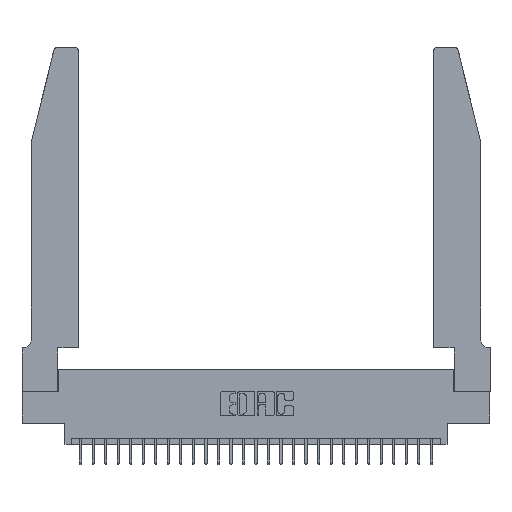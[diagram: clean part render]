
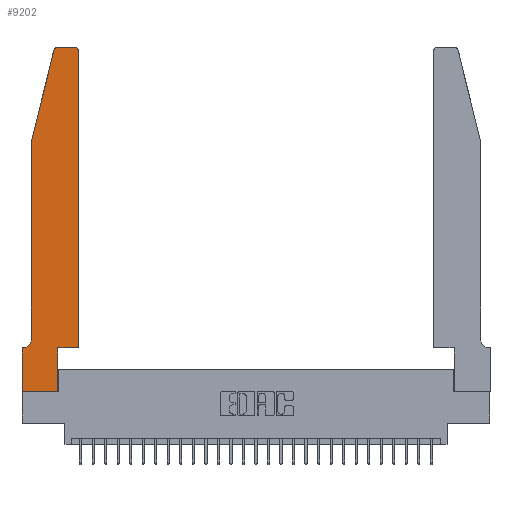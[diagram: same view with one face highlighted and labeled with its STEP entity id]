
A CAD part, top view. The second image highlights one B-rep face of the part: STEP entity #9202.
In plain terms, the highlighted planar face has unit normal (0, 0, 1).
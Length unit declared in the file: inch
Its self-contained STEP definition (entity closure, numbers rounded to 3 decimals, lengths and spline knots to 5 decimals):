
#356 = CARTESIAN_POINT ( 'NONE',  ( 0.4505, 0.35, 0.37 ) ) ;
#701 = CARTESIAN_POINT ( 'NONE',  ( 0.0755, 2., 0.37 ) ) ;
#728 = AXIS2_PLACEMENT_3D ( 'NONE', #21425, #10027, #25942 ) ;
#833 = VECTOR ( 'NONE', #1342, 39.37008 ) ;
#1273 = VECTOR ( 'NONE', #21099, 39.37008 ) ;
#1334 = CARTESIAN_POINT ( 'NONE',  ( 0.4205, 2.75, 0.37 ) ) ;
#1342 = DIRECTION ( 'NONE',  ( 0., -1., 0. ) ) ;
#1542 = EDGE_CURVE ( 'NONE', #26571, #23493, #13890, .T. ) ;
#2296 = EDGE_CURVE ( 'NONE', #9188, #12529, #13505, .T. ) ;
#2359 = ORIENTED_EDGE ( 'NONE', *, *, #21481, .T. ) ;
#2656 = CARTESIAN_POINT ( 'NONE',  ( 0.0755, 0.42, 0.37 ) ) ;
#2674 = CARTESIAN_POINT ( 'NONE',  ( 0.4505, 2.72, 0.37 ) ) ;
#2843 = CARTESIAN_POINT ( 'NONE',  ( 0.0755, 0.35, 0.37 ) ) ;
#2919 = LINE ( 'NONE', #22502, #20438 ) ;
#3110 = DIRECTION ( 'NONE',  ( 0., 1., 0. ) ) ;
#3209 = ORIENTED_EDGE ( 'NONE', *, *, #3962, .T. ) ;
#3780 = ORIENTED_EDGE ( 'NONE', *, *, #15778, .T. ) ;
#3796 = DIRECTION ( 'NONE',  ( -1., 0., 0. ) ) ;
#3881 = DIRECTION ( 'NONE',  ( -0.239, -0.971, 0. ) ) ;
#3962 = EDGE_CURVE ( 'NONE', #12656, #25117, #19539, .T. ) ;
#4898 = VERTEX_POINT ( 'NONE', #7583 ) ;
#5451 = CARTESIAN_POINT ( 'NONE',  ( 0.2865, 0., 0.37 ) ) ;
#6145 = EDGE_CURVE ( 'NONE', #12529, #4898, #19934, .T. ) ;
#6250 = FACE_OUTER_BOUND ( 'NONE', #17310, .T. ) ;
#6573 = DIRECTION ( 'NONE',  ( 0., 0., 1. ) ) ;
#6598 = LINE ( 'NONE', #2843, #18710 ) ;
#6709 = LINE ( 'NONE', #22166, #22785 ) ;
#7068 = VECTOR ( 'NONE', #18686, 39.37008 ) ;
#7450 = CARTESIAN_POINT ( 'NONE',  ( 0.0055, 0.42, 0.37 ) ) ;
#7583 = CARTESIAN_POINT ( 'NONE',  ( 0.4505, 0.35, 0.37 ) ) ;
#7631 = PLANE ( 'NONE',  #728 ) ;
#8285 = CARTESIAN_POINT ( 'NONE',  ( 0.25487, 2.72718, 0.37 ) ) ;
#8880 = EDGE_CURVE ( 'NONE', #13089, #15470, #12637, .T. ) ;
#9188 = VERTEX_POINT ( 'NONE', #5451 ) ;
#9202 = ADVANCED_FACE ( 'NONE', ( #6250 ), #7631, .T. ) ;
#9682 = VECTOR ( 'NONE', #3110, 39.37008 ) ;
#9712 = CARTESIAN_POINT ( 'NONE',  ( 0., 0., 0.37 ) ) ;
#9746 = DIRECTION ( 'NONE',  ( -1., 0., 0. ) ) ;
#9800 = ORIENTED_EDGE ( 'NONE', *, *, #8880, .T. ) ;
#9913 = CARTESIAN_POINT ( 'NONE',  ( 0.4505, 0.35, 0.37 ) ) ;
#9932 = VERTEX_POINT ( 'NONE', #8285 ) ;
#10027 = DIRECTION ( 'NONE',  ( 0., 0., 1. ) ) ;
#10673 = VECTOR ( 'NONE', #3796, 39.37008 ) ;
#10720 = AXIS2_PLACEMENT_3D ( 'NONE', #25015, #11337, #27245 ) ;
#10824 = CARTESIAN_POINT ( 'NONE',  ( 0.284, 2.75, 0.37 ) ) ;
#10858 = EDGE_CURVE ( 'NONE', #4898, #13089, #21123, .T. ) ;
#11337 = DIRECTION ( 'NONE',  ( 0., 0., 1. ) ) ;
#11508 = ORIENTED_EDGE ( 'NONE', *, *, #17144, .T. ) ;
#12090 = ORIENTED_EDGE ( 'NONE', *, *, #2296, .T. ) ;
#12384 = CARTESIAN_POINT ( 'NONE',  ( 0., 0.35, 0.37 ) ) ;
#12529 = VERTEX_POINT ( 'NONE', #14310 ) ;
#12589 = ORIENTED_EDGE ( 'NONE', *, *, #23916, .T. ) ;
#12637 = CIRCLE ( 'NONE', #24861, 0.03 ) ;
#12656 = VERTEX_POINT ( 'NONE', #12384 ) ;
#13023 = LINE ( 'NONE', #26374, #833 ) ;
#13089 = VERTEX_POINT ( 'NONE', #2674 ) ;
#13420 = EDGE_CURVE ( 'NONE', #9932, #27993, #6709, .T. ) ;
#13505 = LINE ( 'NONE', #21193, #18865 ) ;
#13513 = ORIENTED_EDGE ( 'NONE', *, *, #13420, .T. ) ;
#13890 = CIRCLE ( 'NONE', #19588, 0.07 ) ;
#14228 = DIRECTION ( 'NONE',  ( -1., 0., 0. ) ) ;
#14310 = CARTESIAN_POINT ( 'NONE',  ( 0.2865, 0.35, 0.37 ) ) ;
#15470 = VERTEX_POINT ( 'NONE', #1334 ) ;
#15778 = EDGE_CURVE ( 'NONE', #23493, #12656, #6598, .T. ) ;
#16755 = LINE ( 'NONE', #28726, #10673 ) ;
#16785 = DIRECTION ( 'NONE',  ( 0., 1., 0. ) ) ;
#17144 = EDGE_CURVE ( 'NONE', #15470, #29418, #16755, .T. ) ;
#17310 = EDGE_LOOP ( 'NONE', ( #11508, #12589, #13513, #19763, #23486, #3780, #3209, #2359, #12090, #25854, #27426, #9800 ) ) ;
#18686 = DIRECTION ( 'NONE',  ( 1., 0., 0. ) ) ;
#18710 = VECTOR ( 'NONE', #14228, 39.37008 ) ;
#18865 = VECTOR ( 'NONE', #16785, 39.37008 ) ;
#19539 = LINE ( 'NONE', #9712, #1273 ) ;
#19588 = AXIS2_PLACEMENT_3D ( 'NONE', #7450, #23437, #9746 ) ;
#19763 = ORIENTED_EDGE ( 'NONE', *, *, #24259, .T. ) ;
#19934 = LINE ( 'NONE', #356, #7068 ) ;
#20238 = CARTESIAN_POINT ( 'NONE',  ( 0.4205, 2.72, 0.37 ) ) ;
#20438 = VECTOR ( 'NONE', #24748, 39.37008 ) ;
#21099 = DIRECTION ( 'NONE',  ( 0., -1., 0. ) ) ;
#21123 = LINE ( 'NONE', #9913, #9682 ) ;
#21193 = CARTESIAN_POINT ( 'NONE',  ( 0.2865, 0.35, 0.37 ) ) ;
#21283 = CARTESIAN_POINT ( 'NONE',  ( 0.0055, 0.35, 0.37 ) ) ;
#21425 = CARTESIAN_POINT ( 'NONE',  ( 0., 0.35, 0.37 ) ) ;
#21481 = EDGE_CURVE ( 'NONE', #25117, #9188, #2919, .T. ) ;
#21660 = CIRCLE ( 'NONE', #10720, 0.03 ) ;
#22166 = CARTESIAN_POINT ( 'NONE',  ( 0.0755, 2., 0.37 ) ) ;
#22346 = CARTESIAN_POINT ( 'NONE',  ( 0., 0., 0.37 ) ) ;
#22502 = CARTESIAN_POINT ( 'NONE',  ( 0., 0., 0.37 ) ) ;
#22555 = DIRECTION ( 'NONE',  ( 1., 0., 0. ) ) ;
#22785 = VECTOR ( 'NONE', #3881, 39.37008 ) ;
#23437 = DIRECTION ( 'NONE',  ( 0., 0., -1. ) ) ;
#23486 = ORIENTED_EDGE ( 'NONE', *, *, #1542, .T. ) ;
#23493 = VERTEX_POINT ( 'NONE', #21283 ) ;
#23916 = EDGE_CURVE ( 'NONE', #29418, #9932, #21660, .T. ) ;
#24259 = EDGE_CURVE ( 'NONE', #27993, #26571, #13023, .T. ) ;
#24748 = DIRECTION ( 'NONE',  ( 1., 0., 0. ) ) ;
#24861 = AXIS2_PLACEMENT_3D ( 'NONE', #20238, #6573, #22555 ) ;
#25015 = CARTESIAN_POINT ( 'NONE',  ( 0.284, 2.72, 0.37 ) ) ;
#25117 = VERTEX_POINT ( 'NONE', #22346 ) ;
#25854 = ORIENTED_EDGE ( 'NONE', *, *, #6145, .T. ) ;
#25942 = DIRECTION ( 'NONE',  ( 1., 0., 0. ) ) ;
#26374 = CARTESIAN_POINT ( 'NONE',  ( 0.0755, 2., 0.37 ) ) ;
#26571 = VERTEX_POINT ( 'NONE', #2656 ) ;
#27245 = DIRECTION ( 'NONE',  ( 1., 0., 0. ) ) ;
#27426 = ORIENTED_EDGE ( 'NONE', *, *, #10858, .T. ) ;
#27993 = VERTEX_POINT ( 'NONE', #701 ) ;
#28726 = CARTESIAN_POINT ( 'NONE',  ( 0.2605, 2.75, 0.37 ) ) ;
#29418 = VERTEX_POINT ( 'NONE', #10824 ) ;
